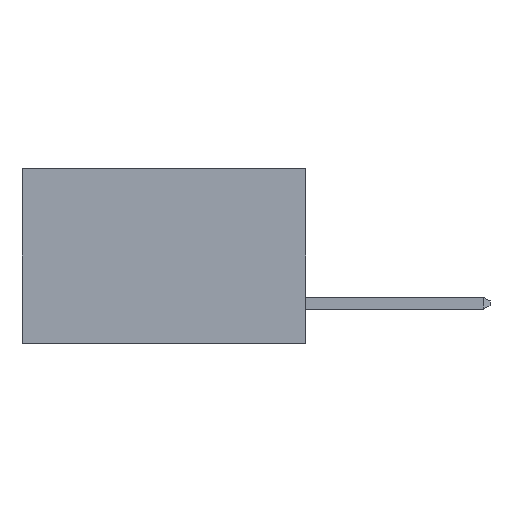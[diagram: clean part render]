
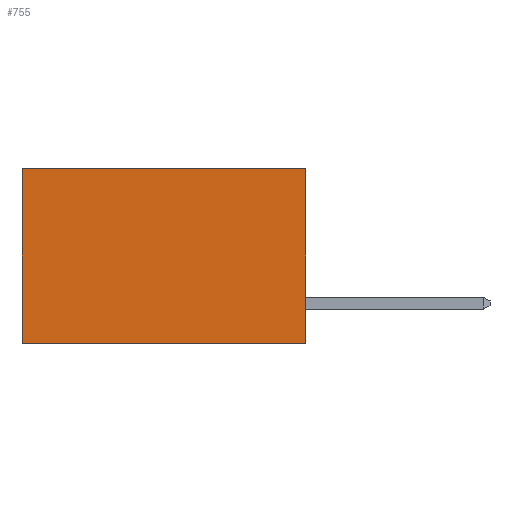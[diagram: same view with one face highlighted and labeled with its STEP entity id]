
A CAD part, left-side view. The second image highlights one B-rep face of the part: STEP entity #755.
In plain terms, the highlighted planar face has unit normal (-1, 0, 0).
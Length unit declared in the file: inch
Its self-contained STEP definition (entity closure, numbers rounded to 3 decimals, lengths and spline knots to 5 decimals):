
#120 = EDGE_LOOP ( 'NONE', ( #8044, #8585, #9889, #3753 ) ) ;
#296 = CARTESIAN_POINT ( 'NONE',  ( 0.298, 0.6, 0. ) ) ;
#364 = LINE ( 'NONE', #490, #7474 ) ;
#446 = VERTEX_POINT ( 'NONE', #296 ) ;
#479 = DIRECTION ( 'NONE',  ( 0., 0., -1. ) ) ;
#490 = CARTESIAN_POINT ( 'NONE',  ( 0.298, 0.6, 0. ) ) ;
#588 = VERTEX_POINT ( 'NONE', #5886 ) ;
#650 = DIRECTION ( 'NONE',  ( 0., 1., 0. ) ) ;
#755 = ADVANCED_FACE ( 'NONE', ( #4084 ), #5324, .F. ) ;
#1264 = VECTOR ( 'NONE', #650, 39.37008 ) ;
#1590 = VERTEX_POINT ( 'NONE', #8717 ) ;
#2659 = VECTOR ( 'NONE', #5773, 39.37008 ) ;
#3031 = VECTOR ( 'NONE', #5365, 39.37008 ) ;
#3209 = AXIS2_PLACEMENT_3D ( 'NONE', #6044, #4422, #10370 ) ;
#3641 = EDGE_CURVE ( 'NONE', #446, #9298, #364, .T. ) ;
#3753 = ORIENTED_EDGE ( 'NONE', *, *, #7214, .T. ) ;
#4084 = FACE_OUTER_BOUND ( 'NONE', #120, .T. ) ;
#4422 = DIRECTION ( 'NONE',  ( 1., 0., 0. ) ) ;
#4974 = LINE ( 'NONE', #8405, #2659 ) ;
#5324 = PLANE ( 'NONE',  #3209 ) ;
#5365 = DIRECTION ( 'NONE',  ( 0., 0., -1. ) ) ;
#5553 = CARTESIAN_POINT ( 'NONE',  ( 0.298, 0., 0. ) ) ;
#5773 = DIRECTION ( 'NONE',  ( 0., 1., 0. ) ) ;
#5886 = CARTESIAN_POINT ( 'NONE',  ( 0.298, 0., 0. ) ) ;
#5993 = LINE ( 'NONE', #5553, #1264 ) ;
#6044 = CARTESIAN_POINT ( 'NONE',  ( 0.298, 0., 0. ) ) ;
#6255 = CARTESIAN_POINT ( 'NONE',  ( 0.298, 0., 0. ) ) ;
#7214 = EDGE_CURVE ( 'NONE', #588, #446, #5993, .T. ) ;
#7474 = VECTOR ( 'NONE', #479, 39.37008 ) ;
#8044 = ORIENTED_EDGE ( 'NONE', *, *, #3641, .T. ) ;
#8405 = CARTESIAN_POINT ( 'NONE',  ( 0.298, 0., -0.37 ) ) ;
#8585 = ORIENTED_EDGE ( 'NONE', *, *, #8966, .F. ) ;
#8717 = CARTESIAN_POINT ( 'NONE',  ( 0.298, 0., -0.37 ) ) ;
#8966 = EDGE_CURVE ( 'NONE', #1590, #9298, #4974, .T. ) ;
#9298 = VERTEX_POINT ( 'NONE', #10572 ) ;
#9889 = ORIENTED_EDGE ( 'NONE', *, *, #9923, .F. ) ;
#9923 = EDGE_CURVE ( 'NONE', #588, #1590, #9967, .T. ) ;
#9967 = LINE ( 'NONE', #6255, #3031 ) ;
#10370 = DIRECTION ( 'NONE',  ( 0., 0., -1. ) ) ;
#10572 = CARTESIAN_POINT ( 'NONE',  ( 0.298, 0.6, -0.37 ) ) ;
